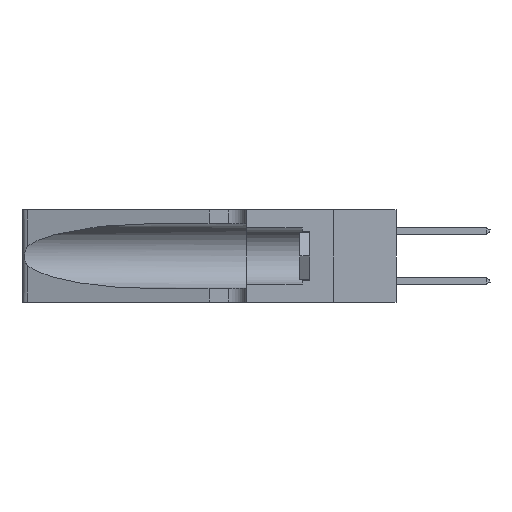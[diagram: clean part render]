
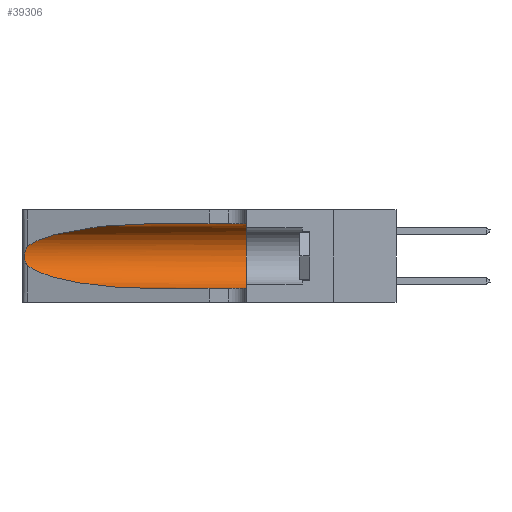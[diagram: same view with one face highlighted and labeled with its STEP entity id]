
A CAD part, left-side view. The second image highlights one B-rep face of the part: STEP entity #39306.
In plain terms, the highlighted cylindrical face has radius 3.308 mm (diameter 6.617 mm), a partial arc.
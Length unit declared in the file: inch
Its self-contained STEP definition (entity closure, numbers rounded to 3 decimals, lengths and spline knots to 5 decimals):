
#1404 = CARTESIAN_POINT ( 'NONE',  ( 0.18966, 0.96281, 0.05475 ) ) ;
#1491 = EDGE_CURVE ( 'NONE', #36956, #28492, #9506, .T. ) ;
#2740 = CARTESIAN_POINT ( 'NONE',  ( 0.25854, 1.2359, 0.20912 ) ) ;
#3074 = ORIENTED_EDGE ( 'NONE', *, *, #17730, .T. ) ;
#3799 = DIRECTION ( 'NONE',  ( 0., 0., 1. ) ) ;
#3866 = DIRECTION ( 'NONE',  ( 0., -1., 0. ) ) ;
#6543 = CARTESIAN_POINT ( 'NONE',  ( 0.26075, 1.23896, 0.19203 ) ) ;
#6582 = VERTEX_POINT ( 'NONE', #20706 ) ;
#7752 = ORIENTED_EDGE ( 'NONE', *, *, #1491, .T. ) ;
#9506 = B_SPLINE_CURVE_WITH_KNOTS ( 'NONE', 3,
 ( #21366, #36149, #43556, #25096, #2740, #28855, #6543, #32597, #10301, #36304, #14028, #40029, #17775, #43710 ),
 .UNSPECIFIED., .F., .F.,
 ( 4, 2, 2, 2, 2, 2, 4 ),
 ( 0., 0.00027, 0.00053, 0.00107, 0.0016, 0.00187, 0.00214 ),
 .UNSPECIFIED. ) ;
#9814 = ORIENTED_EDGE ( 'NONE', *, *, #42385, .F. ) ;
#10127 = CARTESIAN_POINT ( 'NONE',  ( 0.25487, 1.22718, 0.14631 ) ) ;
#10301 = CARTESIAN_POINT ( 'NONE',  ( 0.26017, 1.23833, 0.17102 ) ) ;
#11355 = CARTESIAN_POINT ( 'NONE',  ( 0.1305, 0.35, 0.185 ) ) ;
#11422 = CYLINDRICAL_SURFACE ( 'NONE', #34160, 0.13025 ) ;
#12579 = CARTESIAN_POINT ( 'NONE',  ( 0.2373, 1.15595, 0.08982 ) ) ;
#13716 = LINE ( 'NONE', #28841, #22462 ) ;
#13926 = EDGE_CURVE ( 'NONE', #28492, #42394, #40470, .T. ) ;
#14028 = CARTESIAN_POINT ( 'NONE',  ( 0.25789, 1.23486, 0.15765 ) ) ;
#14287 = CARTESIAN_POINT ( 'NONE',  ( 0.18966, 0.96281, 0.31525 ) ) ;
#15229 = ORIENTED_EDGE ( 'NONE', *, *, #17520, .F. ) ;
#16223 = EDGE_CURVE ( 'NONE', #32002, #36956, #23224, .T. ) ;
#16323 = CARTESIAN_POINT ( 'NONE',  ( 0.1305, 1.61858, 0.185 ) ) ;
#17314 = ORIENTED_EDGE ( 'NONE', *, *, #16223, .T. ) ;
#17520 = EDGE_CURVE ( 'NONE', #32002, #33042, #13716, .T. ) ;
#17730 = EDGE_CURVE ( 'NONE', #42394, #6582, #26516, .T. ) ;
#17775 = CARTESIAN_POINT ( 'NONE',  ( 0.25555, 1.22993, 0.14849 ) ) ;
#17804 = ORIENTED_EDGE ( 'NONE', *, *, #13926, .T. ) ;
#20706 = CARTESIAN_POINT ( 'NONE',  ( 0.1305, 0.35, 0.05475 ) ) ;
#21366 = CARTESIAN_POINT ( 'NONE',  ( 0.25487, 1.22718, 0.22369 ) ) ;
#21389 = CARTESIAN_POINT ( 'NONE',  ( 0.25487, 1.22718, 0.22369 ) ) ;
#22462 = VECTOR ( 'NONE', #32583, 39.37008 ) ;
#23224 =( BOUNDED_CURVE ( )  B_SPLINE_CURVE ( 3, ( #36564, #14287, #47630, #25520 ),
 .UNSPECIFIED., .F., .F. ) 
 B_SPLINE_CURVE_WITH_KNOTS ( ( 4, 4 ),
 ( 1.5708, 2.84003 ),
 .UNSPECIFIED. ) 
 CURVE ( )  GEOMETRIC_REPRESENTATION_ITEM ( )  RATIONAL_B_SPLINE_CURVE ( ( 1., 0.87, 0.87, 1. ) ) 
 REPRESENTATION_ITEM ( '' )  );
#25008 = CARTESIAN_POINT ( 'NONE',  ( 0.1305, 0.35, 0.31525 ) ) ;
#25096 = CARTESIAN_POINT ( 'NONE',  ( 0.25787, 1.23484, 0.2124 ) ) ;
#25520 = CARTESIAN_POINT ( 'NONE',  ( 0.25487, 1.22718, 0.22369 ) ) ;
#26149 = DIRECTION ( 'NONE',  ( 0., 1., 0. ) ) ;
#26516 = LINE ( 'NONE', #29966, #32926 ) ;
#27543 = CARTESIAN_POINT ( 'NONE',  ( 0.1305, 0.72297, 0.05475 ) ) ;
#28492 = VERTEX_POINT ( 'NONE', #10127 ) ;
#28841 = CARTESIAN_POINT ( 'NONE',  ( 0.1305, 1.61858, 0.31525 ) ) ;
#28855 = CARTESIAN_POINT ( 'NONE',  ( 0.26018, 1.23835, 0.19895 ) ) ;
#29900 = CARTESIAN_POINT ( 'NONE',  ( 0.1305, 0.72297, 0.05475 ) ) ;
#29966 = CARTESIAN_POINT ( 'NONE',  ( 0.1305, 1.61858, 0.05475 ) ) ;
#30912 = CIRCLE ( 'NONE', #33304, 0.13025 ) ;
#31233 = FACE_OUTER_BOUND ( 'NONE', #35923, .T. ) ;
#32002 = VERTEX_POINT ( 'NONE', #45308 ) ;
#32583 = DIRECTION ( 'NONE',  ( 0., -1., 0. ) ) ;
#32597 = CARTESIAN_POINT ( 'NONE',  ( 0.26075, 1.23896, 0.178 ) ) ;
#32926 = VECTOR ( 'NONE', #3866, 39.37008 ) ;
#33042 = VERTEX_POINT ( 'NONE', #25008 ) ;
#33304 = AXIS2_PLACEMENT_3D ( 'NONE', #11355, #26149, #3799 ) ;
#34160 = AXIS2_PLACEMENT_3D ( 'NONE', #16323, #34862, #38563 ) ;
#34862 = DIRECTION ( 'NONE',  ( 0., -1., 0. ) ) ;
#35923 = EDGE_LOOP ( 'NONE', ( #17314, #7752, #17804, #3074, #9814, #15229 ) ) ;
#36149 = CARTESIAN_POINT ( 'NONE',  ( 0.25555, 1.22994, 0.2215 ) ) ;
#36304 = CARTESIAN_POINT ( 'NONE',  ( 0.25856, 1.23593, 0.16098 ) ) ;
#36564 = CARTESIAN_POINT ( 'NONE',  ( 0.1305, 0.72297, 0.31525 ) ) ;
#36956 = VERTEX_POINT ( 'NONE', #21389 ) ;
#38558 = CARTESIAN_POINT ( 'NONE',  ( 0.25487, 1.22718, 0.14631 ) ) ;
#38563 = DIRECTION ( 'NONE',  ( 0., 0., -1. ) ) ;
#39306 = ADVANCED_FACE ( 'NONE', ( #31233 ), #11422, .F. ) ;
#40029 = CARTESIAN_POINT ( 'NONE',  ( 0.25639, 1.23186, 0.15144 ) ) ;
#40470 =( BOUNDED_CURVE ( )  B_SPLINE_CURVE ( 3, ( #38558, #12579, #1404, #27543 ),
 .UNSPECIFIED., .F., .T. ) 
 B_SPLINE_CURVE_WITH_KNOTS ( ( 4, 4 ),
 ( 3.44316, 4.71239 ),
 .UNSPECIFIED. ) 
 CURVE ( )  GEOMETRIC_REPRESENTATION_ITEM ( )  RATIONAL_B_SPLINE_CURVE ( ( 1., 0.87, 0.87, 1. ) ) 
 REPRESENTATION_ITEM ( '' )  );
#42385 = EDGE_CURVE ( 'NONE', #33042, #6582, #30912, .T. ) ;
#42394 = VERTEX_POINT ( 'NONE', #29900 ) ;
#43556 = CARTESIAN_POINT ( 'NONE',  ( 0.25639, 1.23184, 0.21858 ) ) ;
#43710 = CARTESIAN_POINT ( 'NONE',  ( 0.25487, 1.22718, 0.14631 ) ) ;
#45308 = CARTESIAN_POINT ( 'NONE',  ( 0.1305, 0.72297, 0.31525 ) ) ;
#47630 = CARTESIAN_POINT ( 'NONE',  ( 0.2373, 1.15595, 0.28018 ) ) ;
